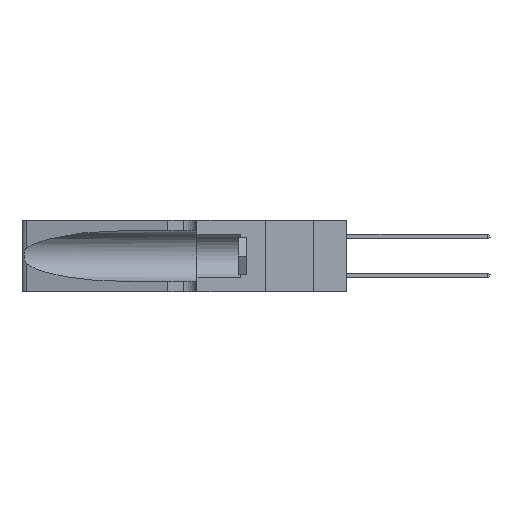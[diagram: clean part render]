
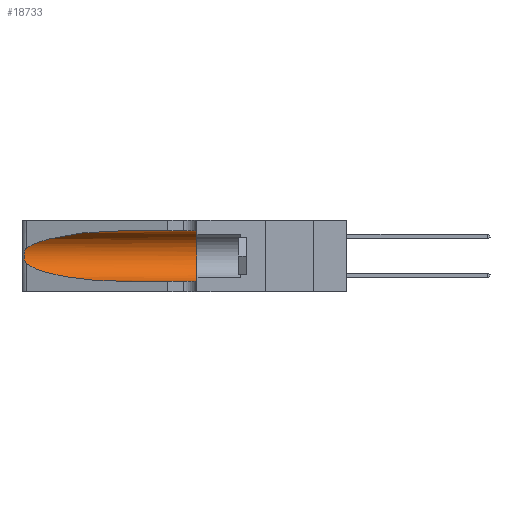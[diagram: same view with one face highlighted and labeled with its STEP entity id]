
A CAD part, left-side view. The second image highlights one B-rep face of the part: STEP entity #18733.
In plain terms, the highlighted cylindrical face has radius 3.308 mm (diameter 6.617 mm), a partial arc.
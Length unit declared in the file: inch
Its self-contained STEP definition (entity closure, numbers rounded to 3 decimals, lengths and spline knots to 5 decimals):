
#229 = EDGE_CURVE ( 'NONE', #16904, #14886, #28048, .T. ) ;
#844 = CARTESIAN_POINT ( 'NONE',  ( 0.25487, 1.22718, 0.14631 ) ) ;
#1242 = CARTESIAN_POINT ( 'NONE',  ( 0.2373, 1.15595, 0.08982 ) ) ;
#1627 = CARTESIAN_POINT ( 'NONE',  ( 0.18966, 0.96281, 0.31525 ) ) ;
#2221 = CARTESIAN_POINT ( 'NONE',  ( 0.26075, 1.23896, 0.178 ) ) ;
#3070 = CARTESIAN_POINT ( 'NONE',  ( 0.1305, 0.35, 0.185 ) ) ;
#3469 = CARTESIAN_POINT ( 'NONE',  ( 0.1305, 1.61858, 0.31525 ) ) ;
#3767 = CARTESIAN_POINT ( 'NONE',  ( 0.1305, 0.72297, 0.05475 ) ) ;
#4743 = CARTESIAN_POINT ( 'NONE',  ( 0.25856, 1.23593, 0.16098 ) ) ;
#5611 = DIRECTION ( 'NONE',  ( 0., 0., 1. ) ) ;
#6096 = ORIENTED_EDGE ( 'NONE', *, *, #13005, .F. ) ;
#7057 = VERTEX_POINT ( 'NONE', #10890 ) ;
#7128 = FACE_OUTER_BOUND ( 'NONE', #12572, .T. ) ;
#7261 = CARTESIAN_POINT ( 'NONE',  ( 0.25639, 1.23186, 0.15144 ) ) ;
#7303 = ORIENTED_EDGE ( 'NONE', *, *, #14817, .T. ) ;
#8195 =( BOUNDED_CURVE ( )  B_SPLINE_CURVE ( 3, ( #24235, #1627, #29226, #14235 ),
 .UNSPECIFIED., .F., .F. ) 
 B_SPLINE_CURVE_WITH_KNOTS ( ( 4, 4 ),
 ( 1.5708, 2.84003 ),
 .UNSPECIFIED. ) 
 CURVE ( )  GEOMETRIC_REPRESENTATION_ITEM ( )  RATIONAL_B_SPLINE_CURVE ( ( 1., 0.87, 0.87, 1. ) ) 
 REPRESENTATION_ITEM ( '' )  );
#9344 = CARTESIAN_POINT ( 'NONE',  ( 0.25487, 1.22718, 0.22369 ) ) ;
#9807 = CARTESIAN_POINT ( 'NONE',  ( 0.25487, 1.22718, 0.14631 ) ) ;
#10890 = CARTESIAN_POINT ( 'NONE',  ( 0.1305, 0.72297, 0.31525 ) ) ;
#11126 = VERTEX_POINT ( 'NONE', #13991 ) ;
#12256 = EDGE_CURVE ( 'NONE', #22948, #11126, #31566, .T. ) ;
#12572 = EDGE_LOOP ( 'NONE', ( #31681, #25748, #19554, #7303, #13372, #6096 ) ) ;
#13005 = EDGE_CURVE ( 'NONE', #7057, #22948, #23722, .T. ) ;
#13114 = CARTESIAN_POINT ( 'NONE',  ( 0.1305, 1.61858, 0.185 ) ) ;
#13144 = CARTESIAN_POINT ( 'NONE',  ( 0.1305, 1.61858, 0.05475 ) ) ;
#13372 = ORIENTED_EDGE ( 'NONE', *, *, #12256, .F. ) ;
#13751 = CARTESIAN_POINT ( 'NONE',  ( 0.25487, 1.22718, 0.14631 ) ) ;
#13991 = CARTESIAN_POINT ( 'NONE',  ( 0.1305, 0.35, 0.05475 ) ) ;
#13992 =( BOUNDED_CURVE ( )  B_SPLINE_CURVE ( 3, ( #13751, #1242, #18798, #3767 ),
 .UNSPECIFIED., .F., .T. ) 
 B_SPLINE_CURVE_WITH_KNOTS ( ( 4, 4 ),
 ( 3.44316, 4.71239 ),
 .UNSPECIFIED. ) 
 CURVE ( )  GEOMETRIC_REPRESENTATION_ITEM ( )  RATIONAL_B_SPLINE_CURVE ( ( 1., 0.87, 0.87, 1. ) ) 
 REPRESENTATION_ITEM ( '' )  );
#14235 = CARTESIAN_POINT ( 'NONE',  ( 0.25487, 1.22718, 0.22369 ) ) ;
#14727 = CARTESIAN_POINT ( 'NONE',  ( 0.25854, 1.2359, 0.20912 ) ) ;
#14817 = EDGE_CURVE ( 'NONE', #23625, #11126, #28669, .T. ) ;
#14864 = CARTESIAN_POINT ( 'NONE',  ( 0.25787, 1.23484, 0.2124 ) ) ;
#14886 = VERTEX_POINT ( 'NONE', #844 ) ;
#15353 = VECTOR ( 'NONE', #15665, 39.37008 ) ;
#15598 = CARTESIAN_POINT ( 'NONE',  ( 0.1305, 0.35, 0.31525 ) ) ;
#15605 = AXIS2_PLACEMENT_3D ( 'NONE', #3070, #20646, #5611 ) ;
#15636 = DIRECTION ( 'NONE',  ( 0., 0., -1. ) ) ;
#15665 = DIRECTION ( 'NONE',  ( 0., -1., 0. ) ) ;
#16904 = VERTEX_POINT ( 'NONE', #9344 ) ;
#17239 = CARTESIAN_POINT ( 'NONE',  ( 0.26075, 1.23896, 0.19203 ) ) ;
#18081 = CARTESIAN_POINT ( 'NONE',  ( 0.1305, 0.72297, 0.05475 ) ) ;
#18733 = ADVANCED_FACE ( 'NONE', ( #7128 ), #32204, .F. ) ;
#18798 = CARTESIAN_POINT ( 'NONE',  ( 0.18966, 0.96281, 0.05475 ) ) ;
#19554 = ORIENTED_EDGE ( 'NONE', *, *, #24505, .T. ) ;
#19787 = CARTESIAN_POINT ( 'NONE',  ( 0.26017, 1.23833, 0.17102 ) ) ;
#20646 = DIRECTION ( 'NONE',  ( 0., 1., 0. ) ) ;
#20706 = DIRECTION ( 'NONE',  ( 0., -1., 0. ) ) ;
#22240 = CARTESIAN_POINT ( 'NONE',  ( 0.25639, 1.23184, 0.21858 ) ) ;
#22303 = CARTESIAN_POINT ( 'NONE',  ( 0.25789, 1.23486, 0.15765 ) ) ;
#22554 = CARTESIAN_POINT ( 'NONE',  ( 0.25487, 1.22718, 0.22369 ) ) ;
#22936 = VECTOR ( 'NONE', #30953, 39.37008 ) ;
#22948 = VERTEX_POINT ( 'NONE', #15598 ) ;
#23625 = VERTEX_POINT ( 'NONE', #18081 ) ;
#23722 = LINE ( 'NONE', #3469, #22936 ) ;
#24235 = CARTESIAN_POINT ( 'NONE',  ( 0.1305, 0.72297, 0.31525 ) ) ;
#24505 = EDGE_CURVE ( 'NONE', #14886, #23625, #13992, .T. ) ;
#24808 = CARTESIAN_POINT ( 'NONE',  ( 0.25555, 1.22993, 0.14849 ) ) ;
#24816 = EDGE_CURVE ( 'NONE', #7057, #16904, #8195, .T. ) ;
#25748 = ORIENTED_EDGE ( 'NONE', *, *, #229, .T. ) ;
#28048 = B_SPLINE_CURVE_WITH_KNOTS ( 'NONE', 3,
 ( #22554, #30542, #22240, #14864, #14727, #32224, #17239, #2221, #19787, #4743, #22303, #7261, #24808, #9807 ),
 .UNSPECIFIED., .F., .F.,
 ( 4, 2, 2, 2, 2, 2, 4 ),
 ( 0., 0.00027, 0.00053, 0.00107, 0.0016, 0.00187, 0.00214 ),
 .UNSPECIFIED. ) ;
#28669 = LINE ( 'NONE', #13144, #15353 ) ;
#29226 = CARTESIAN_POINT ( 'NONE',  ( 0.2373, 1.15595, 0.28018 ) ) ;
#30542 = CARTESIAN_POINT ( 'NONE',  ( 0.25555, 1.22994, 0.2215 ) ) ;
#30953 = DIRECTION ( 'NONE',  ( 0., -1., 0. ) ) ;
#31566 = CIRCLE ( 'NONE', #15605, 0.13025 ) ;
#31681 = ORIENTED_EDGE ( 'NONE', *, *, #24816, .T. ) ;
#32204 = CYLINDRICAL_SURFACE ( 'NONE', #32461, 0.13025 ) ;
#32224 = CARTESIAN_POINT ( 'NONE',  ( 0.26018, 1.23835, 0.19895 ) ) ;
#32461 = AXIS2_PLACEMENT_3D ( 'NONE', #13114, #20706, #15636 ) ;
